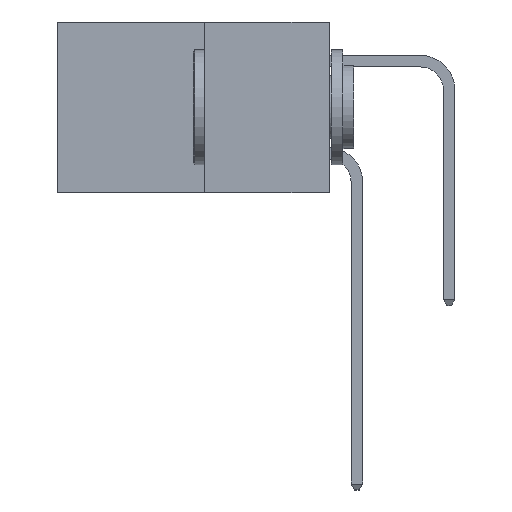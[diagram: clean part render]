
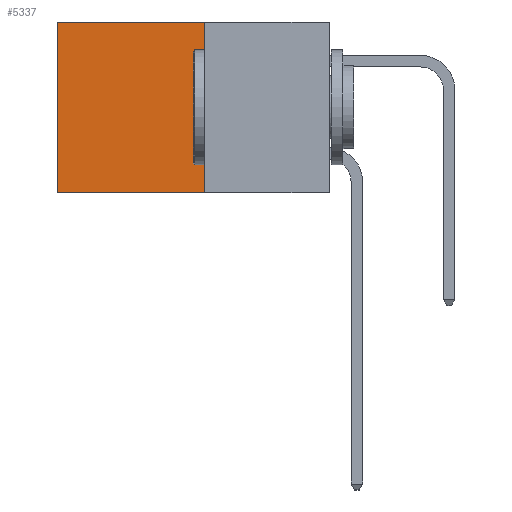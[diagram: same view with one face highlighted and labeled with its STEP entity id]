
A CAD part, left-side view. The second image highlights one B-rep face of the part: STEP entity #5337.
In plain terms, the highlighted planar face has unit normal (-1, 0, 0).
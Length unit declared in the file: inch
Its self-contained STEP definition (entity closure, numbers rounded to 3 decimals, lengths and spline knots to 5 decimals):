
#891 = PLANE ( 'NONE',  #5099 ) ;
#1181 = ORIENTED_EDGE ( 'NONE', *, *, #5753, .T. ) ;
#1515 = CARTESIAN_POINT ( 'NONE',  ( 0.277, 0.27, -0.37 ) ) ;
#1854 = CARTESIAN_POINT ( 'NONE',  ( 0.277, 0.27, 0. ) ) ;
#1947 = DIRECTION ( 'NONE',  ( 0., 1., 0. ) ) ;
#1974 = VECTOR ( 'NONE', #2867, 39.37008 ) ;
#2046 = CARTESIAN_POINT ( 'NONE',  ( 0.277, 0.27, -0.37 ) ) ;
#2267 = LINE ( 'NONE', #1515, #13750 ) ;
#2646 = EDGE_CURVE ( 'NONE', #11875, #5932, #2267, .T. ) ;
#2867 = DIRECTION ( 'NONE',  ( 0., 0., -1. ) ) ;
#3000 = DIRECTION ( 'NONE',  ( 0., 1., 0. ) ) ;
#3679 = CARTESIAN_POINT ( 'NONE',  ( 0.277, 0.27, -0.37 ) ) ;
#3829 = EDGE_LOOP ( 'NONE', ( #1181, #10207, #8009, #8341 ) ) ;
#3994 = CARTESIAN_POINT ( 'NONE',  ( 0.277, 0.59, 0. ) ) ;
#4398 = VECTOR ( 'NONE', #3000, 39.37008 ) ;
#4404 = DIRECTION ( 'NONE',  ( 1., 0., 0. ) ) ;
#5099 = AXIS2_PLACEMENT_3D ( 'NONE', #2046, #4404, #12072 ) ;
#5190 = EDGE_CURVE ( 'NONE', #10420, #10499, #7083, .T. ) ;
#5291 = FACE_OUTER_BOUND ( 'NONE', #3829, .T. ) ;
#5337 = ADVANCED_FACE ( 'NONE', ( #5291 ), #891, .F. ) ;
#5753 = EDGE_CURVE ( 'NONE', #10499, #5932, #8922, .T. ) ;
#5932 = VERTEX_POINT ( 'NONE', #6542 ) ;
#5989 = VECTOR ( 'NONE', #9550, 39.37008 ) ;
#6525 = EDGE_CURVE ( 'NONE', #10420, #11875, #8393, .T. ) ;
#6542 = CARTESIAN_POINT ( 'NONE',  ( 0.277, 0.59, -0.37 ) ) ;
#7083 = LINE ( 'NONE', #1854, #4398 ) ;
#7460 = CARTESIAN_POINT ( 'NONE',  ( 0.277, 0.27, -0.37 ) ) ;
#8009 = ORIENTED_EDGE ( 'NONE', *, *, #6525, .F. ) ;
#8341 = ORIENTED_EDGE ( 'NONE', *, *, #5190, .T. ) ;
#8393 = LINE ( 'NONE', #7460, #1974 ) ;
#8922 = LINE ( 'NONE', #10626, #5989 ) ;
#9550 = DIRECTION ( 'NONE',  ( 0., 0., -1. ) ) ;
#10207 = ORIENTED_EDGE ( 'NONE', *, *, #2646, .F. ) ;
#10420 = VERTEX_POINT ( 'NONE', #10573 ) ;
#10499 = VERTEX_POINT ( 'NONE', #3994 ) ;
#10573 = CARTESIAN_POINT ( 'NONE',  ( 0.277, 0.27, 0. ) ) ;
#10626 = CARTESIAN_POINT ( 'NONE',  ( 0.277, 0.59, -0.37 ) ) ;
#11875 = VERTEX_POINT ( 'NONE', #3679 ) ;
#12072 = DIRECTION ( 'NONE',  ( 0., 0., -1. ) ) ;
#13750 = VECTOR ( 'NONE', #1947, 39.37008 ) ;
